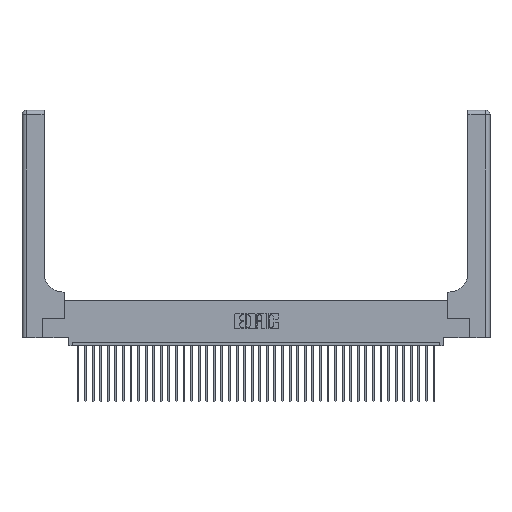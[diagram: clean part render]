
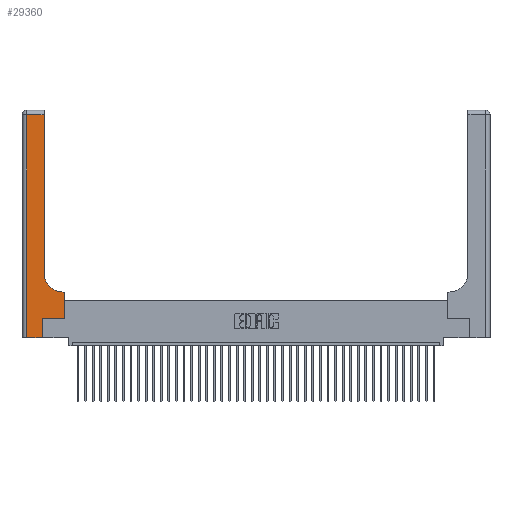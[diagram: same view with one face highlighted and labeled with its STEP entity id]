
A CAD part, top view. The second image highlights one B-rep face of the part: STEP entity #29360.
In plain terms, the highlighted planar face has unit normal (0, 0, 1).
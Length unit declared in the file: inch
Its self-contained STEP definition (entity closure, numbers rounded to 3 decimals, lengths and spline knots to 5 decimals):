
#344 = VECTOR ( 'NONE', #11230, 39.37008 ) ;
#1066 = EDGE_CURVE ( 'NONE', #4753, #31969, #3811, .T. ) ;
#3565 = VECTOR ( 'NONE', #23013, 39.37008 ) ;
#3811 = CIRCLE ( 'NONE', #4247, 0.25 ) ;
#3922 = ORIENTED_EDGE ( 'NONE', *, *, #21506, .T. ) ;
#4247 = AXIS2_PLACEMENT_3D ( 'NONE', #40327, #27649, #15278 ) ;
#4408 = CARTESIAN_POINT ( 'NONE',  ( 0.2915, 3., 0.37 ) ) ;
#4421 = VECTOR ( 'NONE', #18311, 39.37008 ) ;
#4753 = VERTEX_POINT ( 'NONE', #26157 ) ;
#4759 = LINE ( 'NONE', #4408, #6664 ) ;
#4812 = LINE ( 'NONE', #20683, #344 ) ;
#5877 = CARTESIAN_POINT ( 'NONE',  ( 0.06, 3., 0.37 ) ) ;
#6589 = VECTOR ( 'NONE', #22630, 39.37008 ) ;
#6664 = VECTOR ( 'NONE', #35799, 39.37008 ) ;
#6688 = PLANE ( 'NONE',  #26947 ) ;
#7894 = EDGE_CURVE ( 'NONE', #10243, #27136, #9063, .T. ) ;
#8828 = ORIENTED_EDGE ( 'NONE', *, *, #19428, .T. ) ;
#9063 = LINE ( 'NONE', #21047, #10533 ) ;
#9175 = FACE_OUTER_BOUND ( 'NONE', #16295, .T. ) ;
#10243 = VERTEX_POINT ( 'NONE', #15143 ) ;
#10408 = CARTESIAN_POINT ( 'NONE',  ( 0.06, 0., 0.37 ) ) ;
#10533 = VECTOR ( 'NONE', #18327, 39.37008 ) ;
#11230 = DIRECTION ( 'NONE',  ( 0., 1., 0. ) ) ;
#12805 = EDGE_CURVE ( 'NONE', #13276, #37175, #32570, .T. ) ;
#12863 = CARTESIAN_POINT ( 'NONE',  ( 0.06, 2.94, 0.37 ) ) ;
#13276 = VERTEX_POINT ( 'NONE', #10408 ) ;
#13433 = CARTESIAN_POINT ( 'NONE',  ( 0., 0., 0.37 ) ) ;
#14537 = ORIENTED_EDGE ( 'NONE', *, *, #7894, .T. ) ;
#15107 = CARTESIAN_POINT ( 'NONE',  ( 0.2915, 0.85, 0.37 ) ) ;
#15143 = CARTESIAN_POINT ( 'NONE',  ( 0.269, 0.25, 0.37 ) ) ;
#15278 = DIRECTION ( 'NONE',  ( 1., 0., 0. ) ) ;
#15452 = CARTESIAN_POINT ( 'NONE',  ( 0.2915, 0.6, 0.37 ) ) ;
#16295 = EDGE_LOOP ( 'NONE', ( #3922, #8828, #30002, #26193, #22868, #14537, #26561, #39481, #37229 ) ) ;
#18311 = DIRECTION ( 'NONE',  ( -1., 0., 0. ) ) ;
#18327 = DIRECTION ( 'NONE',  ( 1., 0., 0. ) ) ;
#19428 = EDGE_CURVE ( 'NONE', #20602, #36507, #32371, .T. ) ;
#20602 = VERTEX_POINT ( 'NONE', #25449 ) ;
#20683 = CARTESIAN_POINT ( 'NONE',  ( 0.269, 0., 0.37 ) ) ;
#21047 = CARTESIAN_POINT ( 'NONE',  ( 0.269, 0.25, 0.37 ) ) ;
#21506 = EDGE_CURVE ( 'NONE', #31969, #20602, #4759, .T. ) ;
#22236 = VECTOR ( 'NONE', #25768, 39.37008 ) ;
#22590 = DIRECTION ( 'NONE',  ( 0., 0., -1. ) ) ;
#22630 = DIRECTION ( 'NONE',  ( -1., 0., 0. ) ) ;
#22868 = ORIENTED_EDGE ( 'NONE', *, *, #32452, .T. ) ;
#23013 = DIRECTION ( 'NONE',  ( 0., 1., 0. ) ) ;
#23839 = EDGE_CURVE ( 'NONE', #27136, #37031, #34947, .T. ) ;
#24669 = DIRECTION ( 'NONE',  ( 0., -1., 0. ) ) ;
#25133 = CARTESIAN_POINT ( 'NONE',  ( 0.269, 0., 0.37 ) ) ;
#25449 = CARTESIAN_POINT ( 'NONE',  ( 0.2915, 2.94, 0.37 ) ) ;
#25768 = DIRECTION ( 'NONE',  ( 1., 0., 0. ) ) ;
#25913 = DIRECTION ( 'NONE',  ( -1., 0., 0. ) ) ;
#26157 = CARTESIAN_POINT ( 'NONE',  ( 0.5415, 0.6, 0.37 ) ) ;
#26193 = ORIENTED_EDGE ( 'NONE', *, *, #12805, .T. ) ;
#26561 = ORIENTED_EDGE ( 'NONE', *, *, #23839, .T. ) ;
#26947 = AXIS2_PLACEMENT_3D ( 'NONE', #34803, #22590, #25913 ) ;
#27136 = VERTEX_POINT ( 'NONE', #36655 ) ;
#27649 = DIRECTION ( 'NONE',  ( 0., 0., -1. ) ) ;
#27808 = LINE ( 'NONE', #15452, #6589 ) ;
#29360 = ADVANCED_FACE ( 'NONE', ( #9175 ), #6688, .F. ) ;
#30002 = ORIENTED_EDGE ( 'NONE', *, *, #34628, .T. ) ;
#30553 = CARTESIAN_POINT ( 'NONE',  ( 0.5585, 0.6, 0.37 ) ) ;
#31183 = VECTOR ( 'NONE', #24669, 39.37008 ) ;
#31969 = VERTEX_POINT ( 'NONE', #15107 ) ;
#32371 = LINE ( 'NONE', #40476, #4421 ) ;
#32452 = EDGE_CURVE ( 'NONE', #37175, #10243, #4812, .T. ) ;
#32570 = LINE ( 'NONE', #13433, #22236 ) ;
#34628 = EDGE_CURVE ( 'NONE', #36507, #13276, #39500, .T. ) ;
#34803 = CARTESIAN_POINT ( 'NONE',  ( 0., 3., 0.37 ) ) ;
#34947 = LINE ( 'NONE', #39066, #3565 ) ;
#35799 = DIRECTION ( 'NONE',  ( 0., 1., 0. ) ) ;
#36507 = VERTEX_POINT ( 'NONE', #12863 ) ;
#36655 = CARTESIAN_POINT ( 'NONE',  ( 0.5585, 0.25, 0.37 ) ) ;
#37031 = VERTEX_POINT ( 'NONE', #30553 ) ;
#37175 = VERTEX_POINT ( 'NONE', #25133 ) ;
#37229 = ORIENTED_EDGE ( 'NONE', *, *, #1066, .T. ) ;
#38331 = EDGE_CURVE ( 'NONE', #37031, #4753, #27808, .T. ) ;
#39066 = CARTESIAN_POINT ( 'NONE',  ( 0.5585, 0.25, 0.37 ) ) ;
#39481 = ORIENTED_EDGE ( 'NONE', *, *, #38331, .T. ) ;
#39500 = LINE ( 'NONE', #5877, #31183 ) ;
#40327 = CARTESIAN_POINT ( 'NONE',  ( 0.5415, 0.85, 0.37 ) ) ;
#40476 = CARTESIAN_POINT ( 'NONE',  ( 0., 2.94, 0.37 ) ) ;
